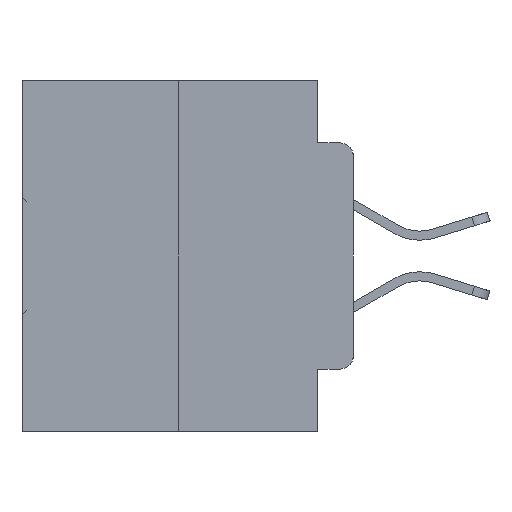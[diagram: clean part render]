
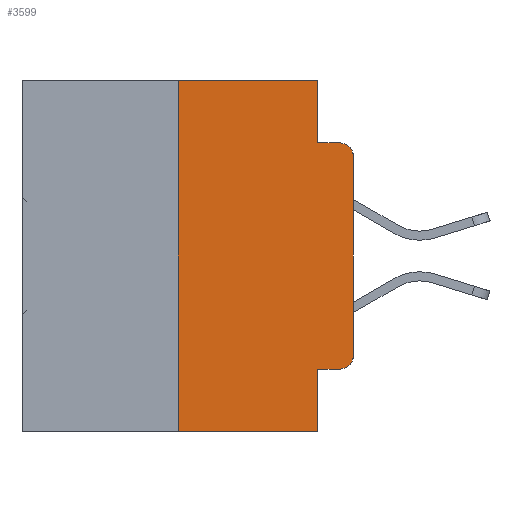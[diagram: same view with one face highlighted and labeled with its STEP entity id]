
A CAD part, left-side view. The second image highlights one B-rep face of the part: STEP entity #3599.
In plain terms, the highlighted planar face has unit normal (-1, 0, 0).
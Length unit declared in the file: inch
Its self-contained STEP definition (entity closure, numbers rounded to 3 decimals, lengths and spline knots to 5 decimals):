
#109 = VERTEX_POINT ( 'NONE', #2275 ) ;
#358 = CARTESIAN_POINT ( 'NONE',  ( 0., 0.02, -0.0885 ) ) ;
#456 = CARTESIAN_POINT ( 'NONE',  ( 0., 0.25, -0.5 ) ) ;
#682 = EDGE_CURVE ( 'NONE', #17243, #5163, #27253, .T. ) ;
#1116 = VECTOR ( 'NONE', #24307, 39.37008 ) ;
#1353 = DIRECTION ( 'NONE',  ( 1., 0., 0. ) ) ;
#1672 = DIRECTION ( 'NONE',  ( -1., 0., 0. ) ) ;
#1688 = LINE ( 'NONE', #5829, #14280 ) ;
#2102 = CARTESIAN_POINT ( 'NONE',  ( 0., 0.051, 0. ) ) ;
#2275 = CARTESIAN_POINT ( 'NONE',  ( 0., 0., -0.1085 ) ) ;
#2483 = VERTEX_POINT ( 'NONE', #15966 ) ;
#2487 = ORIENTED_EDGE ( 'NONE', *, *, #28858, .F. ) ;
#2809 = VERTEX_POINT ( 'NONE', #29473 ) ;
#3135 = CIRCLE ( 'NONE', #18216, 0.02 ) ;
#3357 = VERTEX_POINT ( 'NONE', #358 ) ;
#3415 = DIRECTION ( 'NONE',  ( 0., 0., -1. ) ) ;
#3599 = ADVANCED_FACE ( 'NONE', ( #29023 ), #28576, .F. ) ;
#4450 = CARTESIAN_POINT ( 'NONE',  ( 0., 0.25, 0. ) ) ;
#5163 = VERTEX_POINT ( 'NONE', #17978 ) ;
#5829 = CARTESIAN_POINT ( 'NONE',  ( 0., 0.051, 0. ) ) ;
#6189 = VECTOR ( 'NONE', #16035, 39.37008 ) ;
#6783 = CARTESIAN_POINT ( 'NONE',  ( 0., 0.051, -0.4115 ) ) ;
#7222 = LINE ( 'NONE', #25448, #19774 ) ;
#7981 = AXIS2_PLACEMENT_3D ( 'NONE', #12172, #29747, #14755 ) ;
#8717 = CARTESIAN_POINT ( 'NONE',  ( 0., 0., -0.3915 ) ) ;
#9506 = VERTEX_POINT ( 'NONE', #16976 ) ;
#10326 = ORIENTED_EDGE ( 'NONE', *, *, #16290, .T. ) ;
#10492 = LINE ( 'NONE', #2102, #22301 ) ;
#10642 = CARTESIAN_POINT ( 'NONE',  ( 0., 0.051, 0. ) ) ;
#11425 = CARTESIAN_POINT ( 'NONE',  ( 0., 0.051, -0.0885 ) ) ;
#11620 = ORIENTED_EDGE ( 'NONE', *, *, #29655, .T. ) ;
#11967 = ORIENTED_EDGE ( 'NONE', *, *, #21081, .T. ) ;
#12172 = CARTESIAN_POINT ( 'NONE',  ( 0., 0.02, -0.1085 ) ) ;
#14280 = VECTOR ( 'NONE', #3415, 39.37008 ) ;
#14745 = DIRECTION ( 'NONE',  ( 0., 0., -1. ) ) ;
#14755 = DIRECTION ( 'NONE',  ( 0., 0., -1. ) ) ;
#15130 = AXIS2_PLACEMENT_3D ( 'NONE', #19501, #1353, #26183 ) ;
#15562 = DIRECTION ( 'NONE',  ( 0., 0., 1. ) ) ;
#15921 = ORIENTED_EDGE ( 'NONE', *, *, #26350, .F. ) ;
#15966 = CARTESIAN_POINT ( 'NONE',  ( 0., 0.051, -0.4115 ) ) ;
#16035 = DIRECTION ( 'NONE',  ( 0., -1., 0. ) ) ;
#16079 = VERTEX_POINT ( 'NONE', #8717 ) ;
#16290 = EDGE_CURVE ( 'NONE', #109, #3357, #31001, .T. ) ;
#16419 = VECTOR ( 'NONE', #21544, 39.37008 ) ;
#16730 = CARTESIAN_POINT ( 'NONE',  ( 0., 0.02, -0.3915 ) ) ;
#16976 = CARTESIAN_POINT ( 'NONE',  ( 0., 0.051, -0.0885 ) ) ;
#17206 = LINE ( 'NONE', #11425, #16419 ) ;
#17243 = VERTEX_POINT ( 'NONE', #456 ) ;
#17978 = CARTESIAN_POINT ( 'NONE',  ( 0., 0.25, 0. ) ) ;
#18002 = LINE ( 'NONE', #28526, #6189 ) ;
#18216 = AXIS2_PLACEMENT_3D ( 'NONE', #16730, #1672, #19247 ) ;
#19104 = VERTEX_POINT ( 'NONE', #10642 ) ;
#19247 = DIRECTION ( 'NONE',  ( 0., 0., -1. ) ) ;
#19501 = CARTESIAN_POINT ( 'NONE',  ( 0., 0.473, 0. ) ) ;
#19774 = VECTOR ( 'NONE', #30480, 39.37008 ) ;
#19931 = EDGE_LOOP ( 'NONE', ( #31331, #10326, #15921, #2487, #23386, #26273, #22756, #28871, #11620, #11967 ) ) ;
#20591 = VECTOR ( 'NONE', #15562, 39.37008 ) ;
#20868 = CARTESIAN_POINT ( 'NONE',  ( 0., 0.02, -0.4115 ) ) ;
#21081 = EDGE_CURVE ( 'NONE', #23654, #16079, #3135, .T. ) ;
#21172 = LINE ( 'NONE', #6783, #1116 ) ;
#21544 = DIRECTION ( 'NONE',  ( 0., -1., 0. ) ) ;
#22245 = DIRECTION ( 'NONE',  ( 0., -1., 0. ) ) ;
#22301 = VECTOR ( 'NONE', #14745, 39.37008 ) ;
#22756 = ORIENTED_EDGE ( 'NONE', *, *, #25587, .T. ) ;
#23386 = ORIENTED_EDGE ( 'NONE', *, *, #31141, .F. ) ;
#23654 = VERTEX_POINT ( 'NONE', #20868 ) ;
#24241 = VECTOR ( 'NONE', #22245, 39.37008 ) ;
#24307 = DIRECTION ( 'NONE',  ( 0., -1., 0. ) ) ;
#24656 = CARTESIAN_POINT ( 'NONE',  ( 0., 0.473, 0. ) ) ;
#25220 = EDGE_CURVE ( 'NONE', #2483, #2809, #10492, .T. ) ;
#25448 = CARTESIAN_POINT ( 'NONE',  ( 0., 0., 0. ) ) ;
#25587 = EDGE_CURVE ( 'NONE', #17243, #2809, #18002, .T. ) ;
#26183 = DIRECTION ( 'NONE',  ( 0., 0., -1. ) ) ;
#26273 = ORIENTED_EDGE ( 'NONE', *, *, #682, .F. ) ;
#26350 = EDGE_CURVE ( 'NONE', #9506, #3357, #17206, .T. ) ;
#27253 = LINE ( 'NONE', #4450, #20591 ) ;
#28526 = CARTESIAN_POINT ( 'NONE',  ( 0., 0.473, -0.5 ) ) ;
#28576 = PLANE ( 'NONE',  #15130 ) ;
#28711 = EDGE_CURVE ( 'NONE', #16079, #109, #7222, .T. ) ;
#28858 = EDGE_CURVE ( 'NONE', #19104, #9506, #1688, .T. ) ;
#28871 = ORIENTED_EDGE ( 'NONE', *, *, #25220, .F. ) ;
#29023 = FACE_OUTER_BOUND ( 'NONE', #19931, .T. ) ;
#29473 = CARTESIAN_POINT ( 'NONE',  ( 0., 0.051, -0.5 ) ) ;
#29655 = EDGE_CURVE ( 'NONE', #2483, #23654, #21172, .T. ) ;
#29747 = DIRECTION ( 'NONE',  ( -1., 0., 0. ) ) ;
#30480 = DIRECTION ( 'NONE',  ( 0., 0., 1. ) ) ;
#31001 = CIRCLE ( 'NONE', #7981, 0.02 ) ;
#31141 = EDGE_CURVE ( 'NONE', #5163, #19104, #32419, .T. ) ;
#31331 = ORIENTED_EDGE ( 'NONE', *, *, #28711, .T. ) ;
#32419 = LINE ( 'NONE', #24656, #24241 ) ;
